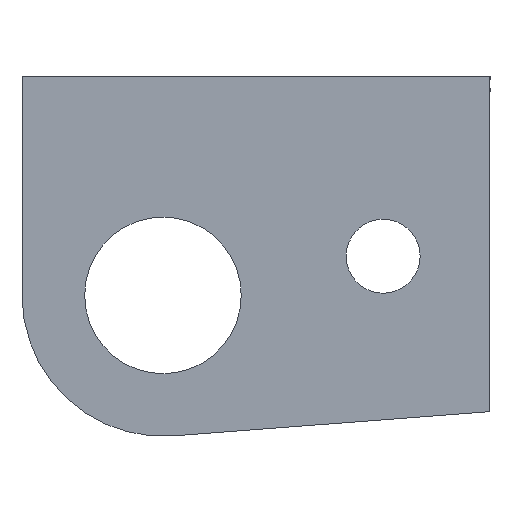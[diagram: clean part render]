
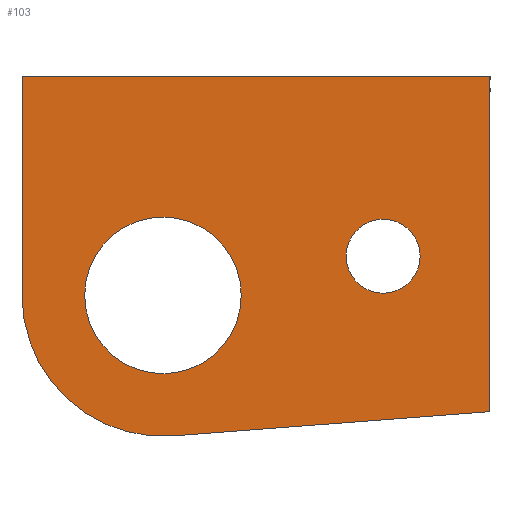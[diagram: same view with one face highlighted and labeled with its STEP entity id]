
A CAD part, left-side view. The second image highlights one B-rep face of the part: STEP entity #103.
In plain terms, the highlighted planar face has unit normal (-1, 0, 0).
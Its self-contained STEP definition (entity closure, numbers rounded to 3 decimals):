
#4 = VERTEX_POINT ( 'NONE', #234 ) ;
#35 = CIRCLE ( 'NONE', #168, 3.175 ) ;
#57 = VECTOR ( 'NONE', #190, 1000. ) ;
#60 = AXIS2_PLACEMENT_3D ( 'NONE', #300, #299, #298 ) ;
#69 = FACE_OUTER_BOUND ( 'NONE', #611, .T. ) ;
#73 = DIRECTION ( 'NONE',  ( 0., 0., -1. ) ) ;
#74 = EDGE_LOOP ( 'NONE', ( #317 ) ) ;
#78 = VECTOR ( 'NONE', #183, 1000. ) ;
#81 = LINE ( 'NONE', #201, #78 ) ;
#83 = DIRECTION ( 'NONE',  ( 1., 0., 0. ) ) ;
#84 = CARTESIAN_POINT ( 'NONE',  ( -11.405, -5.715, 5.715 ) ) ;
#92 = LINE ( 'NONE', #175, #57 ) ;
#103 = ADVANCED_FACE ( 'NONE', ( #641, #209, #69 ), #428, .F. ) ;
#113 = VECTOR ( 'NONE', #245, 1000. ) ;
#114 = LINE ( 'NONE', #254, #113 ) ;
#123 = CARTESIAN_POINT ( 'NONE',  ( -11.405, 0., 14.605 ) ) ;
#131 = AXIS2_PLACEMENT_3D ( 'NONE', #373, #370, #367 ) ;
#159 = CIRCLE ( 'NONE', #60, 1.5 ) ;
#162 = AXIS2_PLACEMENT_3D ( 'NONE', #435, #444, #427 ) ;
#168 = AXIS2_PLACEMENT_3D ( 'NONE', #84, #83, #73 ) ;
#175 = CARTESIAN_POINT ( 'NONE',  ( -11.405, 0., 14.605 ) ) ;
#183 = DIRECTION ( 'NONE',  ( 0., 0.997, -0.076 ) ) ;
#189 = EDGE_CURVE ( 'NONE', #522, #415, #613, .T. ) ;
#190 = DIRECTION ( 'NONE',  ( 0., -1., 0. ) ) ;
#201 = CARTESIAN_POINT ( 'NONE',  ( -11.405, -0.035, -0.452 ) ) ;
#209 = FACE_BOUND ( 'NONE', #74, .T. ) ;
#214 = EDGE_CURVE ( 'NONE', #522, #661, #411, .T. ) ;
#216 = CARTESIAN_POINT ( 'NONE',  ( -11.405, -14.644, 5.802 ) ) ;
#224 = VECTOR ( 'NONE', #403, 1000. ) ;
#234 = CARTESIAN_POINT ( 'NONE',  ( -11.405, -5.715, 2.54 ) ) ;
#245 = DIRECTION ( 'NONE',  ( 0., 0., 1. ) ) ;
#254 = CARTESIAN_POINT ( 'NONE',  ( -11.405, -18.976, 0. ) ) ;
#285 = ORIENTED_EDGE ( 'NONE', *, *, #189, .F. ) ;
#288 = EDGE_CURVE ( 'NONE', #643, #643, #159, .T. ) ;
#292 = CARTESIAN_POINT ( 'NONE',  ( -11.405, 0., 5.715 ) ) ;
#293 = ORIENTED_EDGE ( 'NONE', *, *, #288, .T. ) ;
#294 = CARTESIAN_POINT ( 'NONE',  ( -11.405, -18.976, 0.999 ) ) ;
#298 = DIRECTION ( 'NONE',  ( 0., 0., -1. ) ) ;
#299 = DIRECTION ( 'NONE',  ( 1., 0., 0. ) ) ;
#300 = CARTESIAN_POINT ( 'NONE',  ( -11.405, -14.644, 7.302 ) ) ;
#303 = VERTEX_POINT ( 'NONE', #294 ) ;
#317 = ORIENTED_EDGE ( 'NONE', *, *, #433, .T. ) ;
#327 = EDGE_CURVE ( 'NONE', #303, #593, #114, .T. ) ;
#367 = DIRECTION ( 'NONE',  ( 0., 0., -1. ) ) ;
#368 = EDGE_CURVE ( 'NONE', #303, #661, #81, .T. ) ;
#370 = DIRECTION ( 'NONE',  ( -1., 0., 0. ) ) ;
#373 = CARTESIAN_POINT ( 'NONE',  ( -11.405, -5.715, 5.715 ) ) ;
#386 = EDGE_CURVE ( 'NONE', #415, #593, #92, .T. ) ;
#389 = ORIENTED_EDGE ( 'NONE', *, *, #327, .T. ) ;
#403 = DIRECTION ( 'NONE',  ( 0., 0., 1. ) ) ;
#411 = CIRCLE ( 'NONE', #131, 5.715 ) ;
#413 = CARTESIAN_POINT ( 'NONE',  ( -11.405, 0., 0. ) ) ;
#415 = VERTEX_POINT ( 'NONE', #123 ) ;
#427 = DIRECTION ( 'NONE',  ( 0., 0., -1. ) ) ;
#428 = PLANE ( 'NONE',  #162 ) ;
#433 = EDGE_CURVE ( 'NONE', #4, #4, #35, .T. ) ;
#435 = CARTESIAN_POINT ( 'NONE',  ( -11.405, 0., 0. ) ) ;
#444 = DIRECTION ( 'NONE',  ( 1., 0., 0. ) ) ;
#489 = EDGE_LOOP ( 'NONE', ( #293 ) ) ;
#522 = VERTEX_POINT ( 'NONE', #292 ) ;
#525 = CARTESIAN_POINT ( 'NONE',  ( -11.405, -6.152, 0.017 ) ) ;
#572 = ORIENTED_EDGE ( 'NONE', *, *, #368, .F. ) ;
#593 = VERTEX_POINT ( 'NONE', #667 ) ;
#611 = EDGE_LOOP ( 'NONE', ( #572, #389, #646, #285, #635 ) ) ;
#613 = LINE ( 'NONE', #413, #224 ) ;
#635 = ORIENTED_EDGE ( 'NONE', *, *, #214, .T. ) ;
#641 = FACE_BOUND ( 'NONE', #489, .T. ) ;
#643 = VERTEX_POINT ( 'NONE', #216 ) ;
#646 = ORIENTED_EDGE ( 'NONE', *, *, #386, .F. ) ;
#661 = VERTEX_POINT ( 'NONE', #525 ) ;
#667 = CARTESIAN_POINT ( 'NONE',  ( -11.405, -18.976, 14.605 ) ) ;
